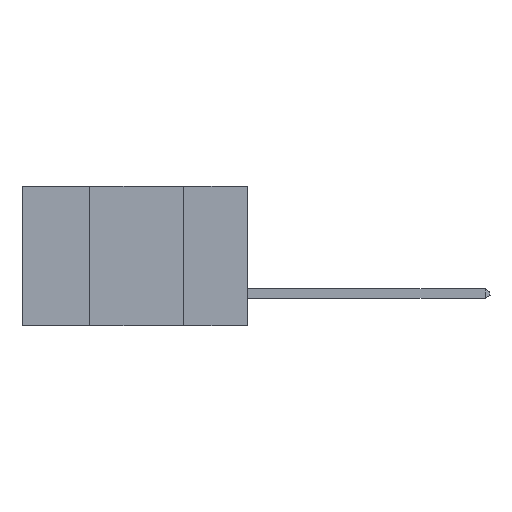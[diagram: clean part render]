
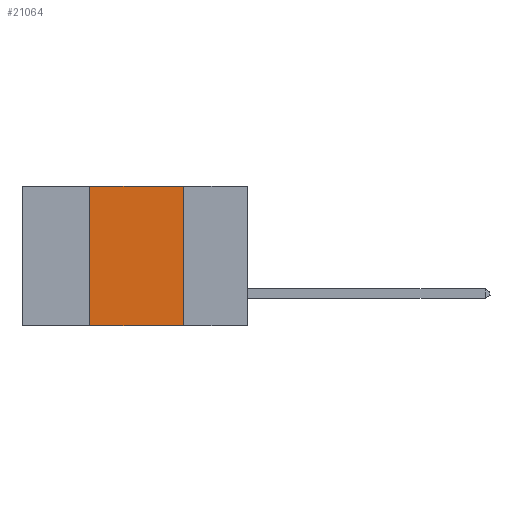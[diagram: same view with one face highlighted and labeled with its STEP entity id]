
A CAD part, left-side view. The second image highlights one B-rep face of the part: STEP entity #21064.
In plain terms, the highlighted planar face has unit normal (-1, 0, 0).
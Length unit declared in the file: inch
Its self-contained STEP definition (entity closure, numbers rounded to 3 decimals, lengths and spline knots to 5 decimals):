
#154 = VECTOR ( 'NONE', #7425, 39.37008 ) ;
#1475 = LINE ( 'NONE', #29221, #7368 ) ;
#2479 = EDGE_CURVE ( 'NONE', #8878, #27930, #1475, .T. ) ;
#3672 = DIRECTION ( 'NONE',  ( 0., -1., 0. ) ) ;
#5162 = AXIS2_PLACEMENT_3D ( 'NONE', #20098, #17695, #20290 ) ;
#5748 = ORIENTED_EDGE ( 'NONE', *, *, #8570, .F. ) ;
#6181 = PLANE ( 'NONE',  #5162 ) ;
#7106 = ORIENTED_EDGE ( 'NONE', *, *, #28483, .T. ) ;
#7368 = VECTOR ( 'NONE', #10132, 39.37008 ) ;
#7425 = DIRECTION ( 'NONE',  ( 0., -1., 0. ) ) ;
#7500 = CARTESIAN_POINT ( 'NONE',  ( 0., 0.42, 0. ) ) ;
#8570 = EDGE_CURVE ( 'NONE', #30716, #8878, #10542, .T. ) ;
#8597 = FACE_OUTER_BOUND ( 'NONE', #22098, .T. ) ;
#8878 = VERTEX_POINT ( 'NONE', #12531 ) ;
#9611 = CARTESIAN_POINT ( 'NONE',  ( 0., 0.42, 0. ) ) ;
#10031 = VECTOR ( 'NONE', #11968, 39.37008 ) ;
#10132 = DIRECTION ( 'NONE',  ( 0., 0., -1. ) ) ;
#10542 = LINE ( 'NONE', #27261, #27952 ) ;
#11968 = DIRECTION ( 'NONE',  ( 0., 0., 1. ) ) ;
#12531 = CARTESIAN_POINT ( 'NONE',  ( 0., 0.17, 0. ) ) ;
#17509 = CARTESIAN_POINT ( 'NONE',  ( 0., 0.17, -0.37 ) ) ;
#17695 = DIRECTION ( 'NONE',  ( 1., 0., 0. ) ) ;
#17715 = VERTEX_POINT ( 'NONE', #29866 ) ;
#20098 = CARTESIAN_POINT ( 'NONE',  ( 0., 0.6, 0. ) ) ;
#20290 = DIRECTION ( 'NONE',  ( 0., 0., -1. ) ) ;
#21064 = ADVANCED_FACE ( 'NONE', ( #8597 ), #6181, .F. ) ;
#21604 = CARTESIAN_POINT ( 'NONE',  ( 0., 0.6, -0.37 ) ) ;
#22098 = EDGE_LOOP ( 'NONE', ( #23356, #5748, #26777, #7106 ) ) ;
#23356 = ORIENTED_EDGE ( 'NONE', *, *, #2479, .F. ) ;
#25137 = EDGE_CURVE ( 'NONE', #17715, #30716, #30442, .T. ) ;
#25324 = LINE ( 'NONE', #21604, #154 ) ;
#26777 = ORIENTED_EDGE ( 'NONE', *, *, #25137, .F. ) ;
#27261 = CARTESIAN_POINT ( 'NONE',  ( 0., 0.6, 0. ) ) ;
#27930 = VERTEX_POINT ( 'NONE', #17509 ) ;
#27952 = VECTOR ( 'NONE', #3672, 39.37008 ) ;
#28483 = EDGE_CURVE ( 'NONE', #17715, #27930, #25324, .T. ) ;
#29221 = CARTESIAN_POINT ( 'NONE',  ( 0., 0.17, 0. ) ) ;
#29866 = CARTESIAN_POINT ( 'NONE',  ( 0., 0.42, -0.37 ) ) ;
#30442 = LINE ( 'NONE', #7500, #10031 ) ;
#30716 = VERTEX_POINT ( 'NONE', #9611 ) ;
